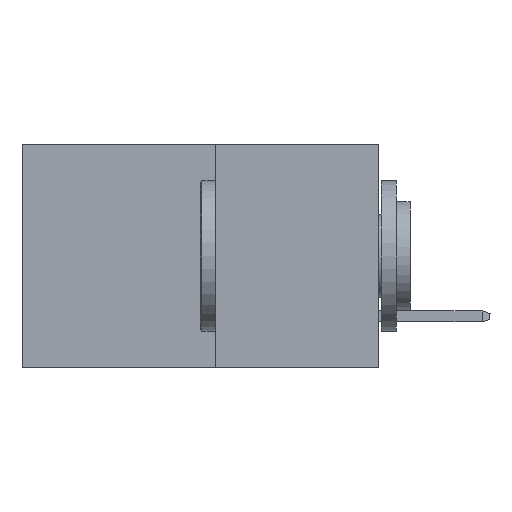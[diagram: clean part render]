
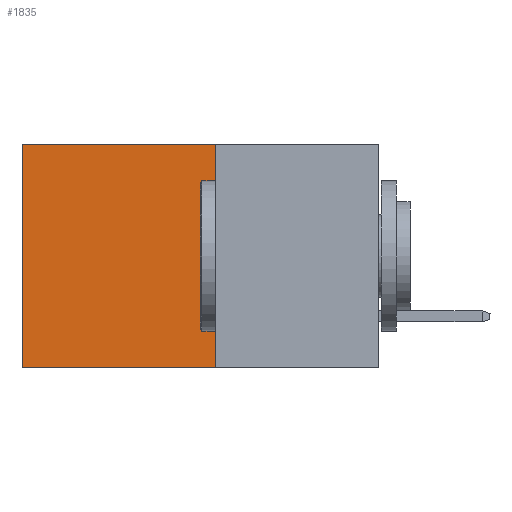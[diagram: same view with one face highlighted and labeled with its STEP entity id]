
A CAD part, left-side view. The second image highlights one B-rep face of the part: STEP entity #1835.
In plain terms, the highlighted planar face has unit normal (-1, 0, 0).
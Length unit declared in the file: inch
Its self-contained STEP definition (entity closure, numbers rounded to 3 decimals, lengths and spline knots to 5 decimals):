
#318 = ORIENTED_EDGE ( 'NONE', *, *, #5793, .T. ) ;
#861 = LINE ( 'NONE', #3618, #4117 ) ;
#1723 = VECTOR ( 'NONE', #15999, 39.37008 ) ;
#1835 = ADVANCED_FACE ( 'NONE', ( #17327 ), #14592, .F. ) ;
#2752 = LINE ( 'NONE', #16072, #1723 ) ;
#2946 = CARTESIAN_POINT ( 'NONE',  ( 0.277, 0.27, 0. ) ) ;
#3216 = EDGE_CURVE ( 'NONE', #10640, #5804, #861, .T. ) ;
#3417 = DIRECTION ( 'NONE',  ( 0., 0., -1. ) ) ;
#3618 = CARTESIAN_POINT ( 'NONE',  ( 0.277, 0.27, -0.37 ) ) ;
#3652 = EDGE_CURVE ( 'NONE', #5804, #19316, #20401, .T. ) ;
#4117 = VECTOR ( 'NONE', #3417, 39.37008 ) ;
#5793 = EDGE_CURVE ( 'NONE', #10640, #15874, #2752, .T. ) ;
#5804 = VERTEX_POINT ( 'NONE', #16136 ) ;
#5823 = AXIS2_PLACEMENT_3D ( 'NONE', #15202, #14413, #14383 ) ;
#8042 = CARTESIAN_POINT ( 'NONE',  ( 0.277, 0.59, -0.37 ) ) ;
#8048 = CARTESIAN_POINT ( 'NONE',  ( 0.277, 0.59, 0. ) ) ;
#8367 = VECTOR ( 'NONE', #15971, 39.37008 ) ;
#9683 = ORIENTED_EDGE ( 'NONE', *, *, #12072, .T. ) ;
#10640 = VERTEX_POINT ( 'NONE', #2946 ) ;
#12065 = VECTOR ( 'NONE', #14907, 39.37008 ) ;
#12072 = EDGE_CURVE ( 'NONE', #15874, #19316, #16797, .T. ) ;
#14383 = DIRECTION ( 'NONE',  ( 0., 0., -1. ) ) ;
#14413 = DIRECTION ( 'NONE',  ( 1., 0., 0. ) ) ;
#14422 = ORIENTED_EDGE ( 'NONE', *, *, #3216, .F. ) ;
#14592 = PLANE ( 'NONE',  #5823 ) ;
#14907 = DIRECTION ( 'NONE',  ( 0., 1., 0. ) ) ;
#15003 = CARTESIAN_POINT ( 'NONE',  ( 0.277, 0.27, -0.37 ) ) ;
#15202 = CARTESIAN_POINT ( 'NONE',  ( 0.277, 0.27, -0.37 ) ) ;
#15874 = VERTEX_POINT ( 'NONE', #8048 ) ;
#15971 = DIRECTION ( 'NONE',  ( 0., 0., -1. ) ) ;
#15999 = DIRECTION ( 'NONE',  ( 0., 1., 0. ) ) ;
#16072 = CARTESIAN_POINT ( 'NONE',  ( 0.277, 0.27, 0. ) ) ;
#16136 = CARTESIAN_POINT ( 'NONE',  ( 0.277, 0.27, -0.37 ) ) ;
#16248 = EDGE_LOOP ( 'NONE', ( #9683, #20317, #14422, #318 ) ) ;
#16797 = LINE ( 'NONE', #8042, #8367 ) ;
#17327 = FACE_OUTER_BOUND ( 'NONE', #16248, .T. ) ;
#19316 = VERTEX_POINT ( 'NONE', #19786 ) ;
#19786 = CARTESIAN_POINT ( 'NONE',  ( 0.277, 0.59, -0.37 ) ) ;
#20317 = ORIENTED_EDGE ( 'NONE', *, *, #3652, .F. ) ;
#20401 = LINE ( 'NONE', #15003, #12065 ) ;
